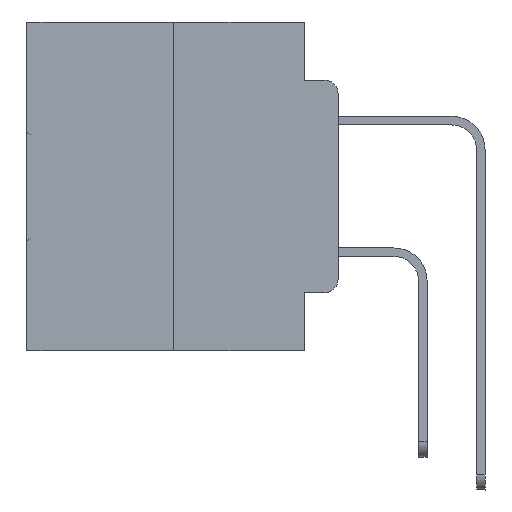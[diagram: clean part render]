
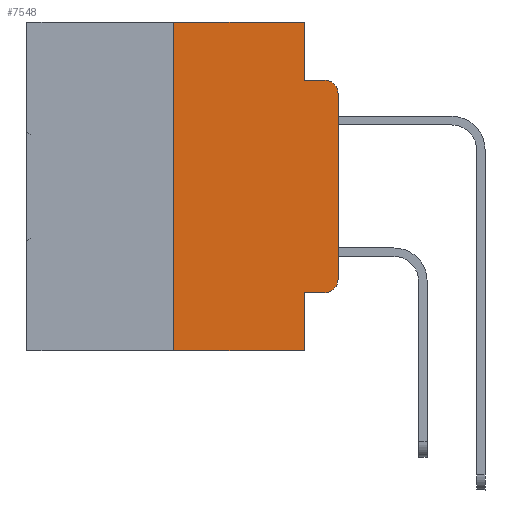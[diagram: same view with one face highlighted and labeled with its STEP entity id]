
A CAD part, left-side view. The second image highlights one B-rep face of the part: STEP entity #7548.
In plain terms, the highlighted planar face has unit normal (-1, 0, 0).
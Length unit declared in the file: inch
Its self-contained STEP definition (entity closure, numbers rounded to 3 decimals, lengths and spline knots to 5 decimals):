
#455 = VECTOR ( 'NONE', #29871, 39.37008 ) ;
#910 = ORIENTED_EDGE ( 'NONE', *, *, #26104, .T. ) ;
#1014 = CARTESIAN_POINT ( 'NONE',  ( 0., 0.473, -0.5 ) ) ;
#1727 = VERTEX_POINT ( 'NONE', #4613 ) ;
#1853 = CARTESIAN_POINT ( 'NONE',  ( 0., 0., -0.1085 ) ) ;
#2094 = VERTEX_POINT ( 'NONE', #23903 ) ;
#2108 = CARTESIAN_POINT ( 'NONE',  ( 0., 0.02, -0.1085 ) ) ;
#2709 = VERTEX_POINT ( 'NONE', #11138 ) ;
#2760 = VECTOR ( 'NONE', #19478, 39.37008 ) ;
#3868 = DIRECTION ( 'NONE',  ( 1., 0., 0. ) ) ;
#3924 = DIRECTION ( 'NONE',  ( 0., -1., 0. ) ) ;
#4047 = PLANE ( 'NONE',  #19577 ) ;
#4613 = CARTESIAN_POINT ( 'NONE',  ( 0., 0.02, -0.0885 ) ) ;
#6839 = VECTOR ( 'NONE', #23743, 39.37008 ) ;
#7184 = VERTEX_POINT ( 'NONE', #14066 ) ;
#7280 = CARTESIAN_POINT ( 'NONE',  ( 0., 0., 0. ) ) ;
#7548 = ADVANCED_FACE ( 'NONE', ( #31458 ), #4047, .F. ) ;
#7765 = ORIENTED_EDGE ( 'NONE', *, *, #13795, .F. ) ;
#7821 = CARTESIAN_POINT ( 'NONE',  ( 0., 0.051, 0. ) ) ;
#7870 = ORIENTED_EDGE ( 'NONE', *, *, #14065, .T. ) ;
#7924 = VERTEX_POINT ( 'NONE', #14408 ) ;
#11085 = VERTEX_POINT ( 'NONE', #22795 ) ;
#11138 = CARTESIAN_POINT ( 'NONE',  ( 0., 0.02, -0.4115 ) ) ;
#11355 = LINE ( 'NONE', #18700, #14526 ) ;
#12280 = DIRECTION ( 'NONE',  ( 0., 0., -1. ) ) ;
#12628 = CARTESIAN_POINT ( 'NONE',  ( 0., 0.051, -0.4115 ) ) ;
#13160 = LINE ( 'NONE', #12628, #6839 ) ;
#13217 = CARTESIAN_POINT ( 'NONE',  ( 0., 0.25, 0. ) ) ;
#13648 = EDGE_CURVE ( 'NONE', #18946, #7924, #21104, .T. ) ;
#13795 = EDGE_CURVE ( 'NONE', #11085, #18946, #30043, .T. ) ;
#13908 = CIRCLE ( 'NONE', #14477, 0.02 ) ;
#14065 = EDGE_CURVE ( 'NONE', #11085, #22587, #25549, .T. ) ;
#14066 = CARTESIAN_POINT ( 'NONE',  ( 0., 0.051, -0.0885 ) ) ;
#14408 = CARTESIAN_POINT ( 'NONE',  ( 0., 0.051, 0. ) ) ;
#14474 = VECTOR ( 'NONE', #26076, 39.37008 ) ;
#14477 = AXIS2_PLACEMENT_3D ( 'NONE', #23860, #34790, #25837 ) ;
#14526 = VECTOR ( 'NONE', #32498, 39.37008 ) ;
#15026 = CARTESIAN_POINT ( 'NONE',  ( 0., 0.473, 0. ) ) ;
#15142 = LINE ( 'NONE', #17488, #21679 ) ;
#16170 = ORIENTED_EDGE ( 'NONE', *, *, #20299, .T. ) ;
#17488 = CARTESIAN_POINT ( 'NONE',  ( 0., 0.051, 0. ) ) ;
#18377 = DIRECTION ( 'NONE',  ( 0., 0., -1. ) ) ;
#18644 = ORIENTED_EDGE ( 'NONE', *, *, #29070, .T. ) ;
#18700 = CARTESIAN_POINT ( 'NONE',  ( 0., 0.051, -0.0885 ) ) ;
#18946 = VERTEX_POINT ( 'NONE', #25230 ) ;
#19061 = CARTESIAN_POINT ( 'NONE',  ( 0., 0.051, -0.4115 ) ) ;
#19478 = DIRECTION ( 'NONE',  ( 0., -1., 0. ) ) ;
#19577 = AXIS2_PLACEMENT_3D ( 'NONE', #33621, #3868, #20346 ) ;
#20299 = EDGE_CURVE ( 'NONE', #2709, #2094, #13908, .T. ) ;
#20346 = DIRECTION ( 'NONE',  ( 0., 0., -1. ) ) ;
#20819 = ORIENTED_EDGE ( 'NONE', *, *, #30862, .F. ) ;
#21087 = CARTESIAN_POINT ( 'NONE',  ( 0., 0.051, -0.5 ) ) ;
#21104 = LINE ( 'NONE', #15026, #25598 ) ;
#21300 = EDGE_CURVE ( 'NONE', #7184, #1727, #11355, .T. ) ;
#21679 = VECTOR ( 'NONE', #12280, 39.37008 ) ;
#21848 = CIRCLE ( 'NONE', #27015, 0.02 ) ;
#22587 = VERTEX_POINT ( 'NONE', #21087 ) ;
#22795 = CARTESIAN_POINT ( 'NONE',  ( 0., 0.25, -0.5 ) ) ;
#23582 = LINE ( 'NONE', #7821, #33351 ) ;
#23743 = DIRECTION ( 'NONE',  ( 0., -1., 0. ) ) ;
#23787 = DIRECTION ( 'NONE',  ( -1., 0., 0. ) ) ;
#23860 = CARTESIAN_POINT ( 'NONE',  ( 0., 0.02, -0.3915 ) ) ;
#23903 = CARTESIAN_POINT ( 'NONE',  ( 0., 0., -0.3915 ) ) ;
#24281 = EDGE_CURVE ( 'NONE', #34005, #22587, #15142, .T. ) ;
#25230 = CARTESIAN_POINT ( 'NONE',  ( 0., 0.25, 0. ) ) ;
#25393 = ORIENTED_EDGE ( 'NONE', *, *, #29677, .T. ) ;
#25549 = LINE ( 'NONE', #1014, #2760 ) ;
#25598 = VECTOR ( 'NONE', #3924, 39.37008 ) ;
#25837 = DIRECTION ( 'NONE',  ( 0., 0., -1. ) ) ;
#26076 = DIRECTION ( 'NONE',  ( 0., 0., 1. ) ) ;
#26104 = EDGE_CURVE ( 'NONE', #34005, #2709, #13160, .T. ) ;
#26382 = ORIENTED_EDGE ( 'NONE', *, *, #21300, .F. ) ;
#26672 = EDGE_LOOP ( 'NONE', ( #25393, #18644, #26382, #20819, #30581, #7765, #7870, #27807, #910, #16170 ) ) ;
#27015 = AXIS2_PLACEMENT_3D ( 'NONE', #2108, #23787, #34898 ) ;
#27807 = ORIENTED_EDGE ( 'NONE', *, *, #24281, .F. ) ;
#29070 = EDGE_CURVE ( 'NONE', #34414, #1727, #21848, .T. ) ;
#29122 = LINE ( 'NONE', #7280, #14474 ) ;
#29677 = EDGE_CURVE ( 'NONE', #2094, #34414, #29122, .T. ) ;
#29871 = DIRECTION ( 'NONE',  ( 0., 0., 1. ) ) ;
#30043 = LINE ( 'NONE', #13217, #455 ) ;
#30581 = ORIENTED_EDGE ( 'NONE', *, *, #13648, .F. ) ;
#30862 = EDGE_CURVE ( 'NONE', #7924, #7184, #23582, .T. ) ;
#31458 = FACE_OUTER_BOUND ( 'NONE', #26672, .T. ) ;
#32498 = DIRECTION ( 'NONE',  ( 0., -1., 0. ) ) ;
#33351 = VECTOR ( 'NONE', #18377, 39.37008 ) ;
#33621 = CARTESIAN_POINT ( 'NONE',  ( 0., 0.473, 0. ) ) ;
#34005 = VERTEX_POINT ( 'NONE', #19061 ) ;
#34414 = VERTEX_POINT ( 'NONE', #1853 ) ;
#34790 = DIRECTION ( 'NONE',  ( -1., 0., 0. ) ) ;
#34898 = DIRECTION ( 'NONE',  ( 0., 0., -1. ) ) ;
